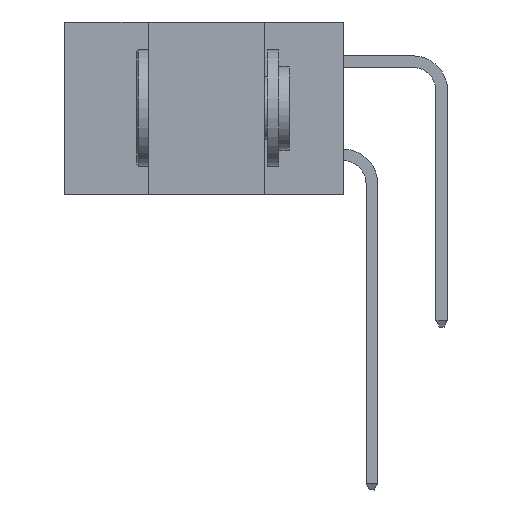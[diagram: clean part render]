
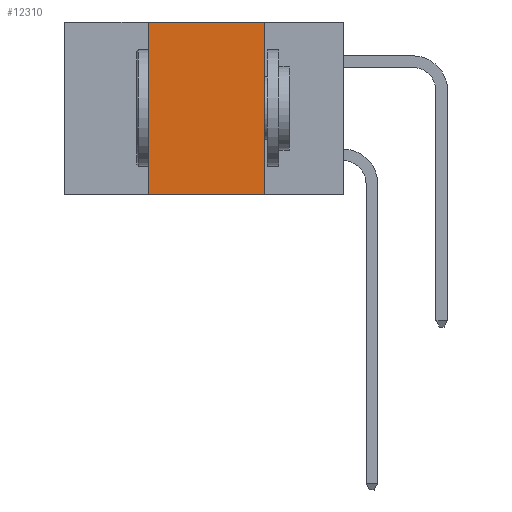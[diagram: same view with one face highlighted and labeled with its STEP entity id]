
A CAD part, left-side view. The second image highlights one B-rep face of the part: STEP entity #12310.
In plain terms, the highlighted planar face has unit normal (-1, 0, 0).
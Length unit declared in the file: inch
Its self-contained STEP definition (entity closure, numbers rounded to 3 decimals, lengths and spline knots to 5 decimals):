
#58 = LINE ( 'NONE', #11710, #7200 ) ;
#709 = EDGE_CURVE ( 'NONE', #1106, #7373, #18040, .T. ) ;
#1106 = VERTEX_POINT ( 'NONE', #17912 ) ;
#1440 = FACE_OUTER_BOUND ( 'NONE', #12604, .T. ) ;
#1686 = DIRECTION ( 'NONE',  ( 0., 0., 1. ) ) ;
#1938 = EDGE_CURVE ( 'NONE', #8141, #18114, #18746, .T. ) ;
#2657 = EDGE_CURVE ( 'NONE', #7373, #8141, #4220, .T. ) ;
#2798 = DIRECTION ( 'NONE',  ( 0., -1., 0. ) ) ;
#3380 = CARTESIAN_POINT ( 'NONE',  ( 0., 0.17, -0.37 ) ) ;
#3577 = CARTESIAN_POINT ( 'NONE',  ( 0., 0.17, -0.37 ) ) ;
#3973 = CARTESIAN_POINT ( 'NONE',  ( 0., 0.42, -0.37 ) ) ;
#4220 = LINE ( 'NONE', #16151, #13646 ) ;
#4693 = DIRECTION ( 'NONE',  ( 0., 0., -1. ) ) ;
#6624 = VECTOR ( 'NONE', #8187, 39.37008 ) ;
#7200 = VECTOR ( 'NONE', #2798, 39.37008 ) ;
#7373 = VERTEX_POINT ( 'NONE', #16947 ) ;
#7820 = ORIENTED_EDGE ( 'NONE', *, *, #1938, .F. ) ;
#8141 = VERTEX_POINT ( 'NONE', #13667 ) ;
#8187 = DIRECTION ( 'NONE',  ( 0., 0., -1. ) ) ;
#8196 = EDGE_CURVE ( 'NONE', #1106, #18114, #58, .T. ) ;
#8979 = CARTESIAN_POINT ( 'NONE',  ( 0., 0.6, 0. ) ) ;
#10380 = DIRECTION ( 'NONE',  ( 0., -1., 0. ) ) ;
#11205 = ORIENTED_EDGE ( 'NONE', *, *, #709, .F. ) ;
#11710 = CARTESIAN_POINT ( 'NONE',  ( 0., 0.6, -0.37 ) ) ;
#12118 = DIRECTION ( 'NONE',  ( 1., 0., 0. ) ) ;
#12310 = ADVANCED_FACE ( 'NONE', ( #1440 ), #16414, .F. ) ;
#12604 = EDGE_LOOP ( 'NONE', ( #7820, #13299, #11205, #12931 ) ) ;
#12931 = ORIENTED_EDGE ( 'NONE', *, *, #8196, .T. ) ;
#13205 = AXIS2_PLACEMENT_3D ( 'NONE', #8979, #12118, #4693 ) ;
#13299 = ORIENTED_EDGE ( 'NONE', *, *, #2657, .F. ) ;
#13646 = VECTOR ( 'NONE', #10380, 39.37008 ) ;
#13667 = CARTESIAN_POINT ( 'NONE',  ( 0., 0.17, 0. ) ) ;
#14213 = VECTOR ( 'NONE', #1686, 39.37008 ) ;
#16151 = CARTESIAN_POINT ( 'NONE',  ( 0., 0.6, 0. ) ) ;
#16414 = PLANE ( 'NONE',  #13205 ) ;
#16947 = CARTESIAN_POINT ( 'NONE',  ( 0., 0.42, 0. ) ) ;
#17912 = CARTESIAN_POINT ( 'NONE',  ( 0., 0.42, -0.37 ) ) ;
#18040 = LINE ( 'NONE', #3973, #14213 ) ;
#18114 = VERTEX_POINT ( 'NONE', #3380 ) ;
#18746 = LINE ( 'NONE', #3577, #6624 ) ;
